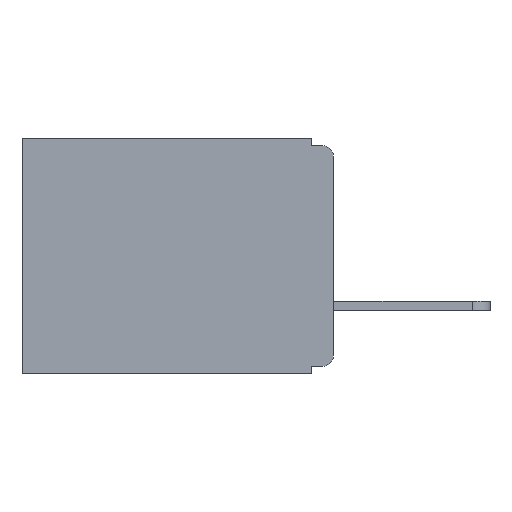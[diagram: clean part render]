
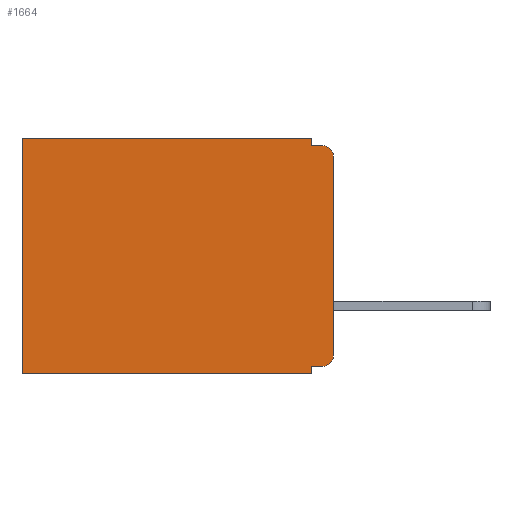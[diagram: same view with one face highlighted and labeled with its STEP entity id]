
A CAD part, left-side view. The second image highlights one B-rep face of the part: STEP entity #1664.
In plain terms, the highlighted planar face has unit normal (-1, 0, 0).
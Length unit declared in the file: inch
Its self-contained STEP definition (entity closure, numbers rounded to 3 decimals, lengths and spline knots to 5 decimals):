
#28 = LINE ( 'NONE', #7581, #615 ) ;
#379 = FACE_OUTER_BOUND ( 'NONE', #11501, .T. ) ;
#615 = VECTOR ( 'NONE', #16355, 39.37008 ) ;
#1127 = DIRECTION ( 'NONE',  ( 1., 0., 0. ) ) ;
#1350 = EDGE_CURVE ( 'NONE', #15252, #12609, #9690, .T. ) ;
#1459 = AXIS2_PLACEMENT_3D ( 'NONE', #6422, #6357, #6341 ) ;
#1513 = VERTEX_POINT ( 'NONE', #2749 ) ;
#1664 = ADVANCED_FACE ( 'NONE', ( #379 ), #11076, .F. ) ;
#2161 = VERTEX_POINT ( 'NONE', #10890 ) ;
#2728 = VECTOR ( 'NONE', #15985, 39.37008 ) ;
#2749 = CARTESIAN_POINT ( 'NONE',  ( 0.3, 0., -0.305 ) ) ;
#2882 = VECTOR ( 'NONE', #7255, 39.37008 ) ;
#2984 = LINE ( 'NONE', #15925, #2728 ) ;
#3445 = CARTESIAN_POINT ( 'NONE',  ( 0.3, 0.031, -0.33 ) ) ;
#3481 = DIRECTION ( 'NONE',  ( -1., 0., 0. ) ) ;
#3570 = VECTOR ( 'NONE', #10516, 39.37008 ) ;
#4183 = CARTESIAN_POINT ( 'NONE',  ( 0.3, 0., -0.33 ) ) ;
#4232 = ORIENTED_EDGE ( 'NONE', *, *, #8388, .T. ) ;
#4705 = LINE ( 'NONE', #13091, #5380 ) ;
#4820 = VERTEX_POINT ( 'NONE', #8906 ) ;
#5104 = VERTEX_POINT ( 'NONE', #8370 ) ;
#5380 = VECTOR ( 'NONE', #13074, 39.37008 ) ;
#6161 = DIRECTION ( 'NONE',  ( 0., 1., 0. ) ) ;
#6341 = DIRECTION ( 'NONE',  ( 0., 0., -1. ) ) ;
#6357 = DIRECTION ( 'NONE',  ( -1., 0., 0. ) ) ;
#6422 = CARTESIAN_POINT ( 'NONE',  ( 0.3, 0.015, -0.025 ) ) ;
#6586 = LINE ( 'NONE', #7082, #2882 ) ;
#6587 = CARTESIAN_POINT ( 'NONE',  ( 0.3, 0.015, -0.32 ) ) ;
#6713 = AXIS2_PLACEMENT_3D ( 'NONE', #9355, #3481, #13347 ) ;
#7051 = CIRCLE ( 'NONE', #6713, 0.015 ) ;
#7082 = CARTESIAN_POINT ( 'NONE',  ( 0.3, 0., -0.01 ) ) ;
#7093 = VERTEX_POINT ( 'NONE', #9956 ) ;
#7255 = DIRECTION ( 'NONE',  ( 0., -1., 0. ) ) ;
#7440 = LINE ( 'NONE', #16270, #13378 ) ;
#7581 = CARTESIAN_POINT ( 'NONE',  ( 0.3, 0., -0.33 ) ) ;
#7781 = ORIENTED_EDGE ( 'NONE', *, *, #16253, .T. ) ;
#8233 = CARTESIAN_POINT ( 'NONE',  ( 0.3, 0.031, -0.33 ) ) ;
#8311 = EDGE_CURVE ( 'NONE', #8524, #1513, #7051, .T. ) ;
#8370 = CARTESIAN_POINT ( 'NONE',  ( 0.3, 0.031, 0. ) ) ;
#8379 = ORIENTED_EDGE ( 'NONE', *, *, #10375, .F. ) ;
#8388 = EDGE_CURVE ( 'NONE', #5104, #11742, #7440, .T. ) ;
#8437 = VECTOR ( 'NONE', #10513, 39.37008 ) ;
#8503 = ORIENTED_EDGE ( 'NONE', *, *, #12022, .F. ) ;
#8524 = VERTEX_POINT ( 'NONE', #6587 ) ;
#8906 = CARTESIAN_POINT ( 'NONE',  ( 0.3, 0., -0.025 ) ) ;
#9008 = ORIENTED_EDGE ( 'NONE', *, *, #9525, .T. ) ;
#9046 = LINE ( 'NONE', #10854, #8437 ) ;
#9068 = CIRCLE ( 'NONE', #1459, 0.015 ) ;
#9355 = CARTESIAN_POINT ( 'NONE',  ( 0.3, 0.015, -0.305 ) ) ;
#9525 = EDGE_CURVE ( 'NONE', #4820, #13254, #9068, .T. ) ;
#9554 = ORIENTED_EDGE ( 'NONE', *, *, #13696, .F. ) ;
#9690 = LINE ( 'NONE', #3445, #3570 ) ;
#9956 = CARTESIAN_POINT ( 'NONE',  ( 0.3, 0.031, -0.01 ) ) ;
#10117 = DIRECTION ( 'NONE',  ( 0., 0., -1. ) ) ;
#10375 = EDGE_CURVE ( 'NONE', #8524, #15252, #2984, .T. ) ;
#10513 = DIRECTION ( 'NONE',  ( 0., 0., -1. ) ) ;
#10516 = DIRECTION ( 'NONE',  ( 0., 0., -1. ) ) ;
#10854 = CARTESIAN_POINT ( 'NONE',  ( 0.3, 0.437, -0.33 ) ) ;
#10890 = CARTESIAN_POINT ( 'NONE',  ( 0.3, 0.437, -0.33 ) ) ;
#11076 = PLANE ( 'NONE',  #12865 ) ;
#11501 = EDGE_LOOP ( 'NONE', ( #8503, #9008, #9554, #16681, #4232, #7781, #14197, #12561, #8379, #12505 ) ) ;
#11742 = VERTEX_POINT ( 'NONE', #16305 ) ;
#12022 = EDGE_CURVE ( 'NONE', #4820, #1513, #13847, .T. ) ;
#12505 = ORIENTED_EDGE ( 'NONE', *, *, #8311, .T. ) ;
#12561 = ORIENTED_EDGE ( 'NONE', *, *, #1350, .F. ) ;
#12609 = VERTEX_POINT ( 'NONE', #8233 ) ;
#12865 = AXIS2_PLACEMENT_3D ( 'NONE', #4183, #1127, #10117 ) ;
#12887 = CARTESIAN_POINT ( 'NONE',  ( 0.3, 0., -0.33 ) ) ;
#12890 = DIRECTION ( 'NONE',  ( 0., 0., -1. ) ) ;
#13074 = DIRECTION ( 'NONE',  ( 0., 0., -1. ) ) ;
#13091 = CARTESIAN_POINT ( 'NONE',  ( 0.3, 0.031, 0. ) ) ;
#13254 = VERTEX_POINT ( 'NONE', #16470 ) ;
#13347 = DIRECTION ( 'NONE',  ( 0., 0., -1. ) ) ;
#13378 = VECTOR ( 'NONE', #6161, 39.37008 ) ;
#13696 = EDGE_CURVE ( 'NONE', #7093, #13254, #6586, .T. ) ;
#13712 = VECTOR ( 'NONE', #12890, 39.37008 ) ;
#13847 = LINE ( 'NONE', #12887, #13712 ) ;
#14197 = ORIENTED_EDGE ( 'NONE', *, *, #14998, .F. ) ;
#14975 = CARTESIAN_POINT ( 'NONE',  ( 0.3, 0.031, -0.32 ) ) ;
#14998 = EDGE_CURVE ( 'NONE', #12609, #2161, #28, .T. ) ;
#15252 = VERTEX_POINT ( 'NONE', #14975 ) ;
#15925 = CARTESIAN_POINT ( 'NONE',  ( 0.3, 0., -0.32 ) ) ;
#15985 = DIRECTION ( 'NONE',  ( 0., 1., 0. ) ) ;
#16253 = EDGE_CURVE ( 'NONE', #11742, #2161, #9046, .T. ) ;
#16270 = CARTESIAN_POINT ( 'NONE',  ( 0.3, 0., 0. ) ) ;
#16305 = CARTESIAN_POINT ( 'NONE',  ( 0.3, 0.437, 0. ) ) ;
#16355 = DIRECTION ( 'NONE',  ( 0., 1., 0. ) ) ;
#16470 = CARTESIAN_POINT ( 'NONE',  ( 0.3, 0.015, -0.01 ) ) ;
#16601 = EDGE_CURVE ( 'NONE', #5104, #7093, #4705, .T. ) ;
#16681 = ORIENTED_EDGE ( 'NONE', *, *, #16601, .F. ) ;
